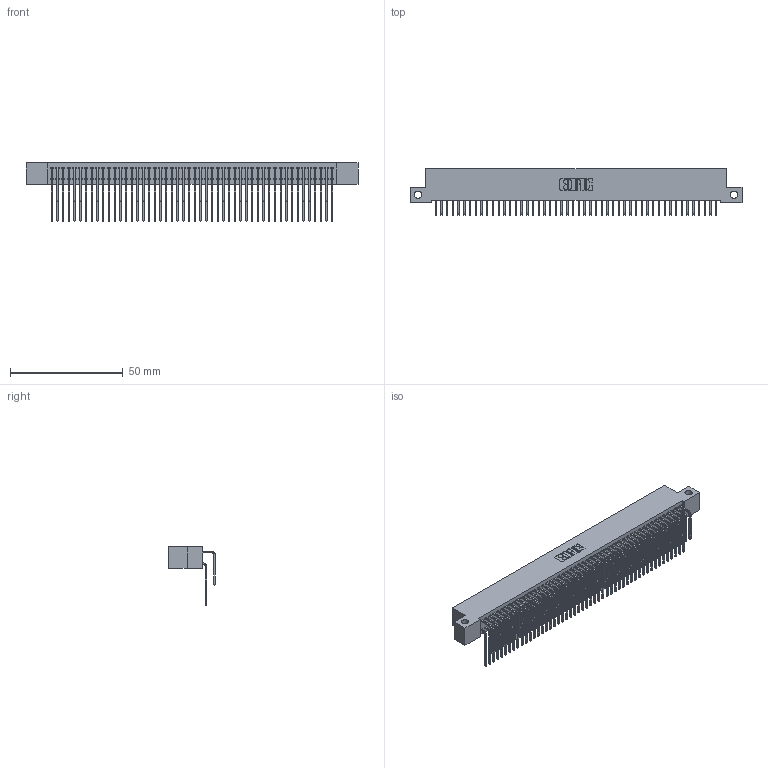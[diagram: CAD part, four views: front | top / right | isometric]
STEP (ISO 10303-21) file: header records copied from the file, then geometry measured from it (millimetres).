
FILE_DESCRIPTION (( 'STEP AP203' ), '1' );
FILE_NAME ('342-100-559-212.STEP', '2018-08-14T04:58:19', ( '' ), ( '' ), 'SwSTEP 2.0', 'SolidWorks 2016', '' );
FILE_SCHEMA (( 'CONFIG_CONTROL_DESIGN' ));
Length unit declared in the file: inch
Products named in the file (4): 342-100-559-212; 342 Part_Side Mount; 345-292-001_558 559 Tail - 1; 345-292-001_559 Tail - 2
Assembly tree (101 placements, depth 2):
  342-100-559-212
    342 Part_Side Mount
    345-292-001_558 559 Tail - 1  x50
    345-292-001_559 Tail - 2  x50
Bounding box: 147.32 x 20.64 x 25.78 mm (x, y, z)
Volume: 13777.5 mm3; surface area: 25073.2 mm2
Topology: 101 solids, 101 shells, 5510 faces, 16399 edges, 10798 vertices
Faces by surface type: plane 3866, cylinder 1644
Entity records: 32787 total; most frequent: CARTESIAN_POINT 5473, ORIENTED_EDGE 5358, DIRECTION 4643, EDGE_CURVE 2679, VECTOR 2511, LINE 2511, VERTEX_POINT 1782, AXIS2_PLACEMENT_3D 1066
